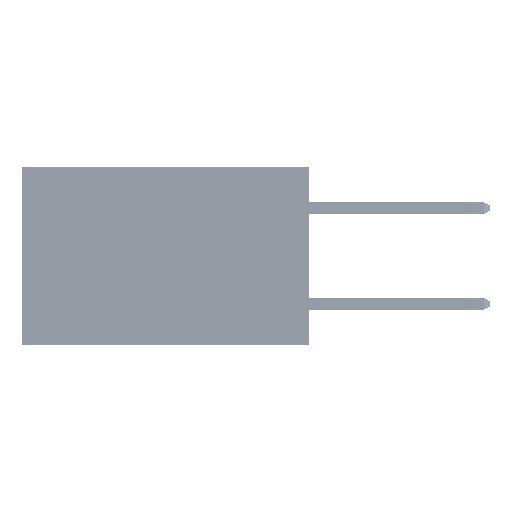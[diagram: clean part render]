
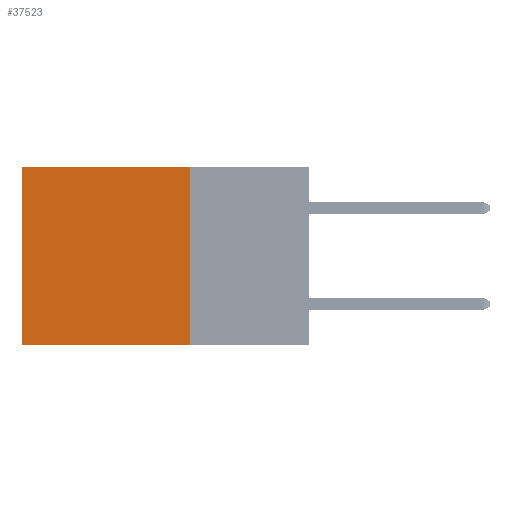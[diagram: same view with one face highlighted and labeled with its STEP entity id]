
A CAD part, left-side view. The second image highlights one B-rep face of the part: STEP entity #37523.
In plain terms, the highlighted planar face has unit normal (-1, 0, 0).
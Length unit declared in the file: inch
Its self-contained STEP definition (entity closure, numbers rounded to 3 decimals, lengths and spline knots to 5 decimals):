
#1009 = VECTOR ( 'NONE', #38683, 39.37008 ) ;
#2320 = VERTEX_POINT ( 'NONE', #8443 ) ;
#2977 = DIRECTION ( 'NONE',  ( 0., 1., 0. ) ) ;
#3012 = EDGE_CURVE ( 'NONE', #41084, #14434, #47802, .T. ) ;
#3791 = DIRECTION ( 'NONE',  ( 1., 0., 0. ) ) ;
#7431 = VECTOR ( 'NONE', #8538, 39.37008 ) ;
#7899 = EDGE_CURVE ( 'NONE', #41084, #40557, #31860, .T. ) ;
#8220 = PLANE ( 'NONE',  #40046 ) ;
#8443 = CARTESIAN_POINT ( 'NONE',  ( 0.2875, 0.6, -0.37 ) ) ;
#8538 = DIRECTION ( 'NONE',  ( 0., 0., -1. ) ) ;
#9170 = EDGE_LOOP ( 'NONE', ( #37614, #22558, #45954, #14455 ) ) ;
#9283 = CARTESIAN_POINT ( 'NONE',  ( 0.2875, 0.25, -0.37 ) ) ;
#14434 = VERTEX_POINT ( 'NONE', #41662 ) ;
#14455 = ORIENTED_EDGE ( 'NONE', *, *, #7899, .T. ) ;
#18087 = CARTESIAN_POINT ( 'NONE',  ( 0.2875, 0.25, 0. ) ) ;
#22558 = ORIENTED_EDGE ( 'NONE', *, *, #39406, .F. ) ;
#22660 = DIRECTION ( 'NONE',  ( 0., 0., -1. ) ) ;
#23131 = CARTESIAN_POINT ( 'NONE',  ( 0.2875, 0.25, 0. ) ) ;
#24045 = DIRECTION ( 'NONE',  ( 0., 1., 0. ) ) ;
#26907 = CARTESIAN_POINT ( 'NONE',  ( 0.2875, 0.25, 0. ) ) ;
#27422 = LINE ( 'NONE', #34830, #1009 ) ;
#31860 = LINE ( 'NONE', #18087, #39422 ) ;
#34830 = CARTESIAN_POINT ( 'NONE',  ( 0.2875, 0.6, 0. ) ) ;
#35077 = VECTOR ( 'NONE', #24045, 39.37008 ) ;
#36403 = FACE_OUTER_BOUND ( 'NONE', #9170, .T. ) ;
#37523 = ADVANCED_FACE ( 'NONE', ( #36403 ), #8220, .F. ) ;
#37614 = ORIENTED_EDGE ( 'NONE', *, *, #48150, .T. ) ;
#38547 = CARTESIAN_POINT ( 'NONE',  ( 0.2875, 0.6, 0. ) ) ;
#38683 = DIRECTION ( 'NONE',  ( 0., 0., -1. ) ) ;
#39406 = EDGE_CURVE ( 'NONE', #14434, #2320, #39713, .T. ) ;
#39422 = VECTOR ( 'NONE', #2977, 39.37008 ) ;
#39713 = LINE ( 'NONE', #9283, #35077 ) ;
#40046 = AXIS2_PLACEMENT_3D ( 'NONE', #45685, #3791, #22660 ) ;
#40557 = VERTEX_POINT ( 'NONE', #38547 ) ;
#41084 = VERTEX_POINT ( 'NONE', #23131 ) ;
#41662 = CARTESIAN_POINT ( 'NONE',  ( 0.2875, 0.25, -0.37 ) ) ;
#45685 = CARTESIAN_POINT ( 'NONE',  ( 0.2875, 0.25, 0. ) ) ;
#45954 = ORIENTED_EDGE ( 'NONE', *, *, #3012, .F. ) ;
#47802 = LINE ( 'NONE', #26907, #7431 ) ;
#48150 = EDGE_CURVE ( 'NONE', #40557, #2320, #27422, .T. ) ;
